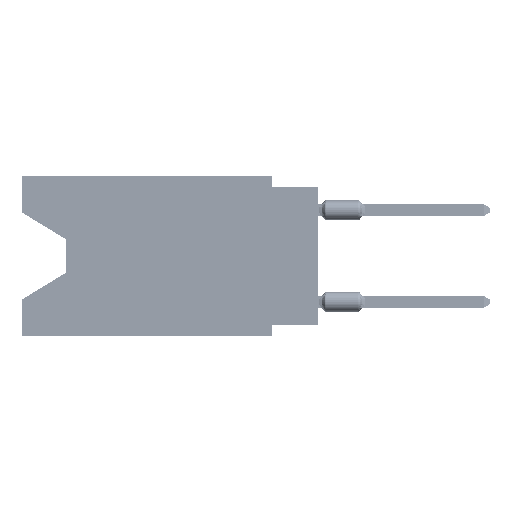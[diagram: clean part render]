
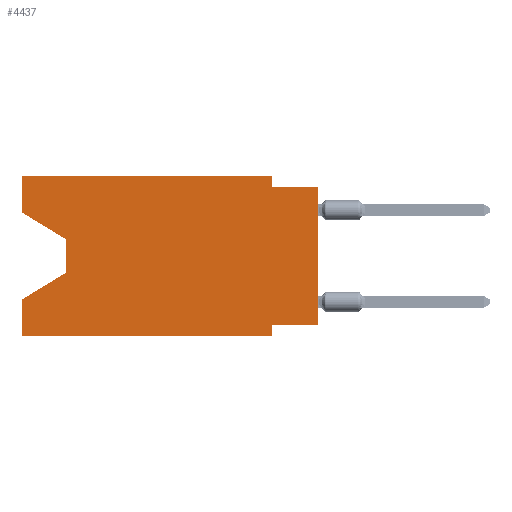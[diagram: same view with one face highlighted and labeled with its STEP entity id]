
A CAD part, left-side view. The second image highlights one B-rep face of the part: STEP entity #4437.
In plain terms, the highlighted planar face has unit normal (-1, 0, 0).
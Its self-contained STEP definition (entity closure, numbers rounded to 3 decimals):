
#1944 = CARTESIAN_POINT ( 'NONE',  ( 0., 2.54, -8.89 ) ) ;
#2540 = EDGE_CURVE ( 'NONE', #39634, #96531, #92381, .T. ) ;
#2800 = CARTESIAN_POINT ( 'NONE',  ( 0., 0., -8.255 ) ) ;
#4034 = DIRECTION ( 'NONE',  ( 0., 0., 1. ) ) ;
#4160 = ORIENTED_EDGE ( 'NONE', *, *, #2540, .F. ) ;
#4437 = ADVANCED_FACE ( 'NONE', ( #47749 ), #32083, .F. ) ;
#7889 = EDGE_CURVE ( 'NONE', #41518, #96531, #82291, .T. ) ;
#7953 = LINE ( 'NONE', #66872, #40993 ) ;
#8159 = LINE ( 'NONE', #68057, #95846 ) ;
#8800 = VERTEX_POINT ( 'NONE', #77950 ) ;
#9799 = VECTOR ( 'NONE', #4034, 1000. ) ;
#9858 = EDGE_CURVE ( 'NONE', #69081, #42607, #7953, .T. ) ;
#11707 = CARTESIAN_POINT ( 'NONE',  ( 0., 16.383, 0. ) ) ;
#11884 = ORIENTED_EDGE ( 'NONE', *, *, #65677, .F. ) ;
#13621 = VECTOR ( 'NONE', #60689, 1000. ) ;
#14071 = DIRECTION ( 'NONE',  ( 0., 1., 0. ) ) ;
#15173 = VERTEX_POINT ( 'NONE', #2800 ) ;
#15534 = DIRECTION ( 'NONE',  ( 0., 0., 1. ) ) ;
#16112 = DIRECTION ( 'NONE',  ( 0., -1., 0. ) ) ;
#16299 = VECTOR ( 'NONE', #71495, 1000. ) ;
#16530 = ORIENTED_EDGE ( 'NONE', *, *, #46349, .T. ) ;
#16537 = EDGE_CURVE ( 'NONE', #15173, #76436, #82780, .T. ) ;
#17665 = CARTESIAN_POINT ( 'NONE',  ( 0., 0., -0.635 ) ) ;
#19691 = EDGE_CURVE ( 'NONE', #42607, #8800, #28925, .T. ) ;
#24013 = ORIENTED_EDGE ( 'NONE', *, *, #83115, .F. ) ;
#24805 = VECTOR ( 'NONE', #16112, 1000. ) ;
#25664 = VECTOR ( 'NONE', #48624, 1000. ) ;
#28925 = LINE ( 'NONE', #38216, #24805 ) ;
#28973 = ORIENTED_EDGE ( 'NONE', *, *, #16537, .T. ) ;
#29131 = CARTESIAN_POINT ( 'NONE',  ( 0., 13.97, -3.505 ) ) ;
#32000 = ORIENTED_EDGE ( 'NONE', *, *, #39724, .F. ) ;
#32083 = PLANE ( 'NONE',  #35258 ) ;
#32691 = ORIENTED_EDGE ( 'NONE', *, *, #50990, .F. ) ;
#33923 = CARTESIAN_POINT ( 'NONE',  ( 0., 13.97, -3.505 ) ) ;
#35258 = AXIS2_PLACEMENT_3D ( 'NONE', #62002, #92399, #84092 ) ;
#35807 = LINE ( 'NONE', #65739, #71146 ) ;
#35859 = EDGE_CURVE ( 'NONE', #39634, #83185, #54844, .T. ) ;
#36904 = VERTEX_POINT ( 'NONE', #96599 ) ;
#38216 = CARTESIAN_POINT ( 'NONE',  ( 0., 16.383, 0. ) ) ;
#39146 = CARTESIAN_POINT ( 'NONE',  ( 0., 16.383, -8.89 ) ) ;
#39634 = VERTEX_POINT ( 'NONE', #94040 ) ;
#39724 = EDGE_CURVE ( 'NONE', #36904, #83185, #45905, .T. ) ;
#40993 = VECTOR ( 'NONE', #67363, 1000. ) ;
#41518 = VERTEX_POINT ( 'NONE', #83599 ) ;
#42027 = EDGE_LOOP ( 'NONE', ( #71019, #16530, #81031, #4160, #44301, #32000, #11884, #28973, #24013, #32691, #43454, #92267 ) ) ;
#42043 = CARTESIAN_POINT ( 'NONE',  ( 0., 2.54, 0. ) ) ;
#42607 = VERTEX_POINT ( 'NONE', #11707 ) ;
#43454 = ORIENTED_EDGE ( 'NONE', *, *, #19691, .F. ) ;
#44301 = ORIENTED_EDGE ( 'NONE', *, *, #35859, .T. ) ;
#45553 = DIRECTION ( 'NONE',  ( 0., -1., 0. ) ) ;
#45905 = LINE ( 'NONE', #67550, #86193 ) ;
#46349 = EDGE_CURVE ( 'NONE', #81268, #41518, #49590, .T. ) ;
#46571 = VECTOR ( 'NONE', #86340, 1000. ) ;
#47749 = FACE_OUTER_BOUND ( 'NONE', #42027, .T. ) ;
#48624 = DIRECTION ( 'NONE',  ( 0., 0., -1. ) ) ;
#49590 = LINE ( 'NONE', #33923, #25664 ) ;
#49715 = CARTESIAN_POINT ( 'NONE',  ( 0., 16.383, -6.852 ) ) ;
#50217 = VECTOR ( 'NONE', #45553, 1000. ) ;
#50677 = CARTESIAN_POINT ( 'NONE',  ( 0., 0., -0.635 ) ) ;
#50990 = EDGE_CURVE ( 'NONE', #8800, #59437, #78382, .T. ) ;
#51344 = DIRECTION ( 'NONE',  ( 0., 0., -1. ) ) ;
#54844 = LINE ( 'NONE', #39146, #50217 ) ;
#58029 = CARTESIAN_POINT ( 'NONE',  ( 0., 16.383, -2.038 ) ) ;
#59437 = VERTEX_POINT ( 'NONE', #72123 ) ;
#60689 = DIRECTION ( 'NONE',  ( 0., 0.855, -0.519 ) ) ;
#62002 = CARTESIAN_POINT ( 'NONE',  ( 0., 16.383, 0. ) ) ;
#64270 = DIRECTION ( 'NONE',  ( 0., -0.855, -0.519 ) ) ;
#65677 = EDGE_CURVE ( 'NONE', #15173, #36904, #8159, .T. ) ;
#65739 = CARTESIAN_POINT ( 'NONE',  ( 0., 16.383, -2.038 ) ) ;
#66872 = CARTESIAN_POINT ( 'NONE',  ( 0., 16.383, 0. ) ) ;
#67363 = DIRECTION ( 'NONE',  ( 0., 0., 1. ) ) ;
#67550 = CARTESIAN_POINT ( 'NONE',  ( 0., 2.54, -8.89 ) ) ;
#67667 = EDGE_CURVE ( 'NONE', #69081, #81268, #35807, .T. ) ;
#68057 = CARTESIAN_POINT ( 'NONE',  ( 0., 0., -8.255 ) ) ;
#68530 = CARTESIAN_POINT ( 'NONE',  ( 0., 0., 0. ) ) ;
#69081 = VERTEX_POINT ( 'NONE', #58029 ) ;
#71019 = ORIENTED_EDGE ( 'NONE', *, *, #67667, .T. ) ;
#71146 = VECTOR ( 'NONE', #64270, 1000. ) ;
#71495 = DIRECTION ( 'NONE',  ( 0., 0., -1. ) ) ;
#72123 = CARTESIAN_POINT ( 'NONE',  ( 0., 2.54, -0.635 ) ) ;
#76436 = VERTEX_POINT ( 'NONE', #50677 ) ;
#77685 = CARTESIAN_POINT ( 'NONE',  ( 0., 16.383, 0. ) ) ;
#77950 = CARTESIAN_POINT ( 'NONE',  ( 0., 2.54, 0. ) ) ;
#78027 = LINE ( 'NONE', #17665, #46571 ) ;
#78382 = LINE ( 'NONE', #42043, #16299 ) ;
#79178 = VECTOR ( 'NONE', #15534, 1000. ) ;
#81031 = ORIENTED_EDGE ( 'NONE', *, *, #7889, .T. ) ;
#81268 = VERTEX_POINT ( 'NONE', #29131 ) ;
#82291 = LINE ( 'NONE', #96991, #13621 ) ;
#82780 = LINE ( 'NONE', #68530, #79178 ) ;
#83115 = EDGE_CURVE ( 'NONE', #59437, #76436, #78027, .T. ) ;
#83185 = VERTEX_POINT ( 'NONE', #1944 ) ;
#83599 = CARTESIAN_POINT ( 'NONE',  ( 0., 13.97, -5.385 ) ) ;
#84092 = DIRECTION ( 'NONE',  ( 0., 0., -1. ) ) ;
#86193 = VECTOR ( 'NONE', #51344, 1000. ) ;
#86340 = DIRECTION ( 'NONE',  ( 0., -1., 0. ) ) ;
#92267 = ORIENTED_EDGE ( 'NONE', *, *, #9858, .F. ) ;
#92381 = LINE ( 'NONE', #77685, #9799 ) ;
#92399 = DIRECTION ( 'NONE',  ( 1., 0., 0. ) ) ;
#94040 = CARTESIAN_POINT ( 'NONE',  ( 0., 16.383, -8.89 ) ) ;
#95846 = VECTOR ( 'NONE', #14071, 1000. ) ;
#96531 = VERTEX_POINT ( 'NONE', #49715 ) ;
#96599 = CARTESIAN_POINT ( 'NONE',  ( 0., 2.54, -8.255 ) ) ;
#96991 = CARTESIAN_POINT ( 'NONE',  ( 0., 13.97, -5.385 ) ) ;
